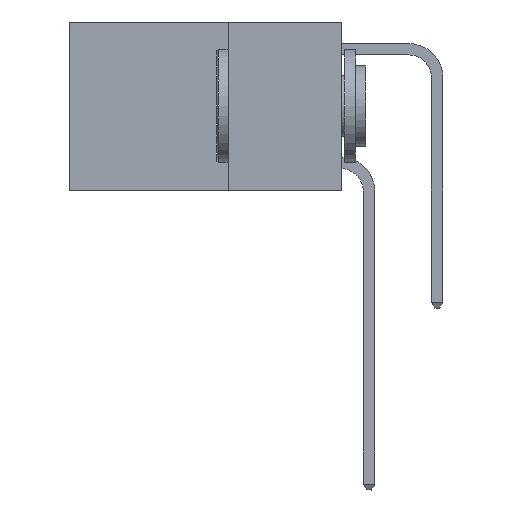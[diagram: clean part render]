
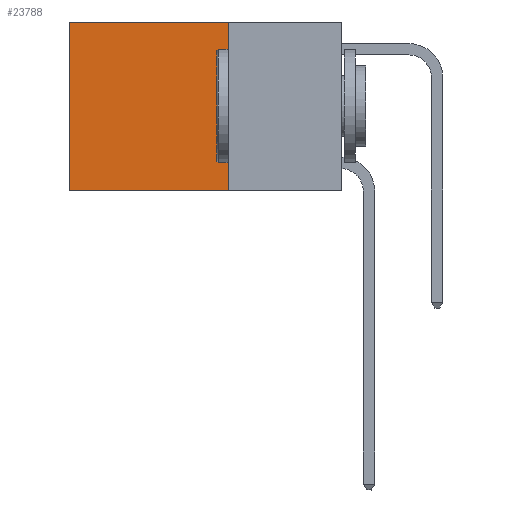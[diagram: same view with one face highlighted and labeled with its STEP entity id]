
A CAD part, left-side view. The second image highlights one B-rep face of the part: STEP entity #23788.
In plain terms, the highlighted planar face has unit normal (-1, 0, 0).
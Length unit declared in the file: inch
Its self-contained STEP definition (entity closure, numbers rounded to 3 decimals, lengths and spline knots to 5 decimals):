
#528 = EDGE_CURVE ( 'NONE', #7068, #21673, #23312, .T. ) ;
#872 = CARTESIAN_POINT ( 'NONE',  ( 0.2625, 0.25, 0. ) ) ;
#1487 = EDGE_CURVE ( 'NONE', #7922, #7068, #21836, .T. ) ;
#2875 = CARTESIAN_POINT ( 'NONE',  ( 0.2625, 0.25, 0. ) ) ;
#3095 = CARTESIAN_POINT ( 'NONE',  ( 0.2625, 0.25, -0.37 ) ) ;
#3142 = LINE ( 'NONE', #872, #21439 ) ;
#4856 = ORIENTED_EDGE ( 'NONE', *, *, #528, .T. ) ;
#4875 = FACE_OUTER_BOUND ( 'NONE', #24276, .T. ) ;
#5517 = CARTESIAN_POINT ( 'NONE',  ( 0.2625, 0.6, -0.37 ) ) ;
#5963 = CARTESIAN_POINT ( 'NONE',  ( 0.2625, 0.25, 0. ) ) ;
#7068 = VERTEX_POINT ( 'NONE', #7910 ) ;
#7910 = CARTESIAN_POINT ( 'NONE',  ( 0.2625, 0.6, 0. ) ) ;
#7922 = VERTEX_POINT ( 'NONE', #2875 ) ;
#8830 = DIRECTION ( 'NONE',  ( 0., 1., 0. ) ) ;
#9292 = LINE ( 'NONE', #18494, #9810 ) ;
#9678 = VECTOR ( 'NONE', #15663, 39.37008 ) ;
#9810 = VECTOR ( 'NONE', #8830, 39.37008 ) ;
#11092 = VECTOR ( 'NONE', #12160, 39.37008 ) ;
#11716 = CARTESIAN_POINT ( 'NONE',  ( 0.2625, 0.6, 0. ) ) ;
#12160 = DIRECTION ( 'NONE',  ( 0., 0., -1. ) ) ;
#13755 = ORIENTED_EDGE ( 'NONE', *, *, #24391, .F. ) ;
#14128 = PLANE ( 'NONE',  #26611 ) ;
#14424 = ORIENTED_EDGE ( 'NONE', *, *, #28359, .F. ) ;
#14434 = VERTEX_POINT ( 'NONE', #3095 ) ;
#14987 = ORIENTED_EDGE ( 'NONE', *, *, #1487, .T. ) ;
#15663 = DIRECTION ( 'NONE',  ( 0., 1., 0. ) ) ;
#17199 = DIRECTION ( 'NONE',  ( 0., 0., -1. ) ) ;
#18494 = CARTESIAN_POINT ( 'NONE',  ( 0.2625, 0.25, -0.37 ) ) ;
#18763 = DIRECTION ( 'NONE',  ( 0., 0., -1. ) ) ;
#21439 = VECTOR ( 'NONE', #17199, 39.37008 ) ;
#21673 = VERTEX_POINT ( 'NONE', #5517 ) ;
#21836 = LINE ( 'NONE', #5963, #9678 ) ;
#23279 = CARTESIAN_POINT ( 'NONE',  ( 0.2625, 0.25, 0. ) ) ;
#23312 = LINE ( 'NONE', #11716, #11092 ) ;
#23788 = ADVANCED_FACE ( 'NONE', ( #4875 ), #14128, .F. ) ;
#24276 = EDGE_LOOP ( 'NONE', ( #4856, #13755, #14424, #14987 ) ) ;
#24391 = EDGE_CURVE ( 'NONE', #14434, #21673, #9292, .T. ) ;
#26611 = AXIS2_PLACEMENT_3D ( 'NONE', #23279, #27809, #18763 ) ;
#27809 = DIRECTION ( 'NONE',  ( 1., 0., 0. ) ) ;
#28359 = EDGE_CURVE ( 'NONE', #7922, #14434, #3142, .T. ) ;
